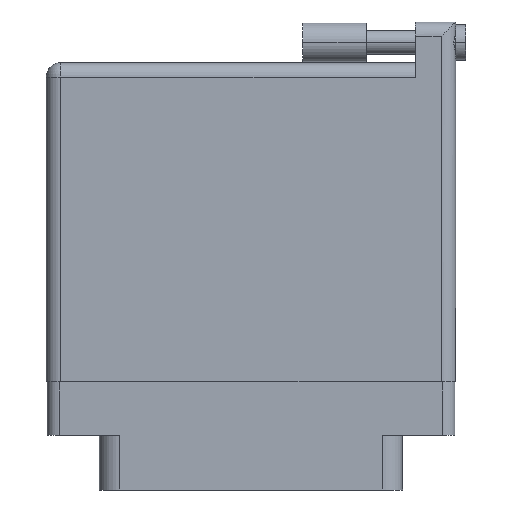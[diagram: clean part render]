
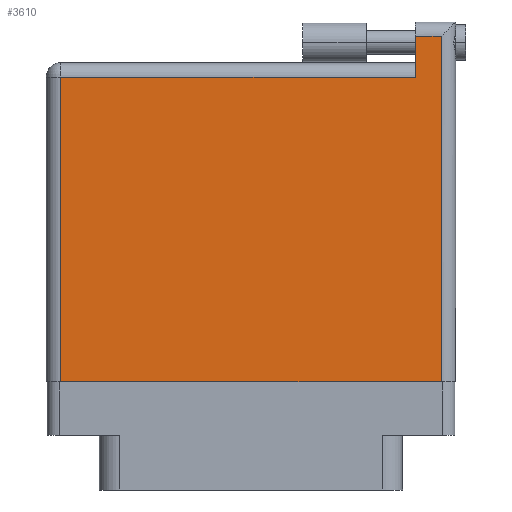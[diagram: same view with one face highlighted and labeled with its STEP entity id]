
A CAD part, front view. The second image highlights one B-rep face of the part: STEP entity #3610.
In plain terms, the highlighted face is planar.
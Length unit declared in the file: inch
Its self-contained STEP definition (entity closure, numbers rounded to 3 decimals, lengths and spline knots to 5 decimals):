
#36 = EDGE_CURVE ( 'NONE', #32562, #6287, #24084, .T. ) ;
#653 = AXIS2_PLACEMENT_3D ( 'NONE', #1535, #30588, #33398 ) ;
#1535 = CARTESIAN_POINT ( 'NONE',  ( 0., 1.566, 0. ) ) ;
#1600 = LINE ( 'NONE', #23122, #28410 ) ;
#2194 = LINE ( 'NONE', #2905, #22715 ) ;
#2905 = CARTESIAN_POINT ( 'NONE',  ( 0., 1.496, 0. ) ) ;
#3366 = EDGE_CURVE ( 'NONE', #14024, #34639, #20594, .T. ) ;
#3610 = ADVANCED_FACE ( 'NONE', ( #24297 ), #17152, .F. ) ;
#4670 = ORIENTED_EDGE ( 'NONE', *, *, #31064, .T. ) ;
#6207 = CARTESIAN_POINT ( 'NONE',  ( 1.811, 1.696, 0. ) ) ;
#6270 = ORIENTED_EDGE ( 'NONE', *, *, #23898, .T. ) ;
#6287 = VERTEX_POINT ( 'NONE', #28788 ) ;
#6703 = VECTOR ( 'NONE', #25483, 39.37008 ) ;
#6939 = ORIENTED_EDGE ( 'NONE', *, *, #3366, .T. ) ;
#8254 = ORIENTED_EDGE ( 'NONE', *, *, #36, .T. ) ;
#9707 = CARTESIAN_POINT ( 'NONE',  ( 0., 0., 0. ) ) ;
#12572 = LINE ( 'NONE', #9707, #6703 ) ;
#13908 = EDGE_CURVE ( 'NONE', #34639, #32562, #20952, .T. ) ;
#13917 = VECTOR ( 'NONE', #27925, 39.37008 ) ;
#14024 = VERTEX_POINT ( 'NONE', #16582 ) ;
#14740 = CARTESIAN_POINT ( 'NONE',  ( 1.811, 1.766, 0. ) ) ;
#15825 = ORIENTED_EDGE ( 'NONE', *, *, #28960, .T. ) ;
#16582 = CARTESIAN_POINT ( 'NONE',  ( 1.938, 0., 0. ) ) ;
#17152 = PLANE ( 'NONE',  #653 ) ;
#17421 = CARTESIAN_POINT ( 'NONE',  ( 1.938, 1.766, 0. ) ) ;
#18858 = VECTOR ( 'NONE', #20882, 39.37008 ) ;
#20594 = LINE ( 'NONE', #17421, #13917 ) ;
#20882 = DIRECTION ( 'NONE',  ( -1., 0., 0. ) ) ;
#20952 = LINE ( 'NONE', #23312, #18858 ) ;
#22375 = CARTESIAN_POINT ( 'NONE',  ( 0.07, 1.496, 0. ) ) ;
#22715 = VECTOR ( 'NONE', #29848, 39.37008 ) ;
#23122 = CARTESIAN_POINT ( 'NONE',  ( 0.07, 0., 0. ) ) ;
#23312 = CARTESIAN_POINT ( 'NONE',  ( 0., 1.696, 0. ) ) ;
#23898 = EDGE_CURVE ( 'NONE', #26850, #14024, #12572, .T. ) ;
#24084 = LINE ( 'NONE', #14740, #32516 ) ;
#24297 = FACE_OUTER_BOUND ( 'NONE', #25446, .T. ) ;
#24416 = CARTESIAN_POINT ( 'NONE',  ( 0.07, 0., 0. ) ) ;
#25446 = EDGE_LOOP ( 'NONE', ( #6270, #6939, #29707, #8254, #15825, #4670 ) ) ;
#25483 = DIRECTION ( 'NONE',  ( 1., 0., 0. ) ) ;
#25595 = DIRECTION ( 'NONE',  ( 0., -1., 0. ) ) ;
#25855 = CARTESIAN_POINT ( 'NONE',  ( 1.938, 1.696, 0. ) ) ;
#26235 = VERTEX_POINT ( 'NONE', #22375 ) ;
#26850 = VERTEX_POINT ( 'NONE', #24416 ) ;
#27925 = DIRECTION ( 'NONE',  ( 0., 1., 0. ) ) ;
#28410 = VECTOR ( 'NONE', #25595, 39.37008 ) ;
#28514 = DIRECTION ( 'NONE',  ( 0., -1., 0. ) ) ;
#28788 = CARTESIAN_POINT ( 'NONE',  ( 1.811, 1.496, 0. ) ) ;
#28960 = EDGE_CURVE ( 'NONE', #6287, #26235, #2194, .T. ) ;
#29707 = ORIENTED_EDGE ( 'NONE', *, *, #13908, .T. ) ;
#29848 = DIRECTION ( 'NONE',  ( -1., 0., 0. ) ) ;
#30588 = DIRECTION ( 'NONE',  ( 0., 0., -1. ) ) ;
#31064 = EDGE_CURVE ( 'NONE', #26235, #26850, #1600, .T. ) ;
#32516 = VECTOR ( 'NONE', #28514, 39.37008 ) ;
#32562 = VERTEX_POINT ( 'NONE', #6207 ) ;
#33398 = DIRECTION ( 'NONE',  ( -1., 0., 0. ) ) ;
#34639 = VERTEX_POINT ( 'NONE', #25855 ) ;
